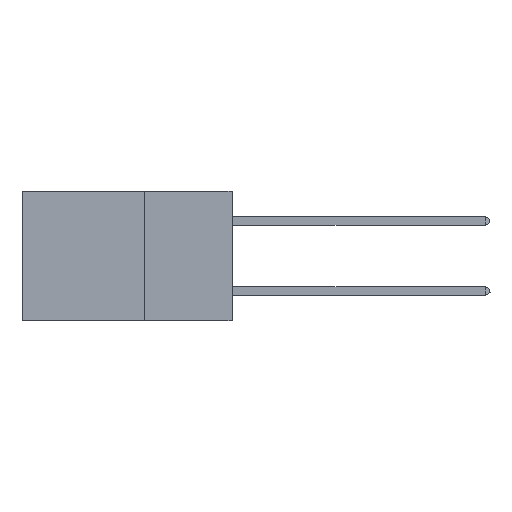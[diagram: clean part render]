
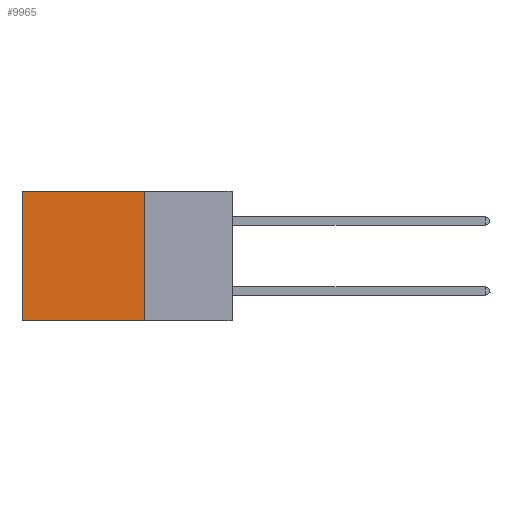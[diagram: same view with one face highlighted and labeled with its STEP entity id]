
A CAD part, left-side view. The second image highlights one B-rep face of the part: STEP entity #9965.
In plain terms, the highlighted planar face has unit normal (-1, 0, 0).
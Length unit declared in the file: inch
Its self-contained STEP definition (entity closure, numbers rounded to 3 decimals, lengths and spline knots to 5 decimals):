
#2030 = CARTESIAN_POINT ( 'NONE',  ( 0.2875, 0.25, -0.37 ) ) ;
#3394 = EDGE_CURVE ( 'NONE', #20159, #12420, #3566, .T. ) ;
#3555 = CARTESIAN_POINT ( 'NONE',  ( 0.2875, 0.25, 0. ) ) ;
#3566 = LINE ( 'NONE', #12758, #24923 ) ;
#4373 = EDGE_CURVE ( 'NONE', #9347, #28542, #22340, .T. ) ;
#5568 = VECTOR ( 'NONE', #29239, 39.37008 ) ;
#5815 = EDGE_CURVE ( 'NONE', #28542, #12420, #25143, .T. ) ;
#6469 = FACE_OUTER_BOUND ( 'NONE', #14280, .T. ) ;
#7150 = LINE ( 'NONE', #3555, #11040 ) ;
#9347 = VERTEX_POINT ( 'NONE', #26755 ) ;
#9965 = ADVANCED_FACE ( 'NONE', ( #6469 ), #13038, .F. ) ;
#10123 = DIRECTION ( 'NONE',  ( 0., 0., -1. ) ) ;
#11040 = VECTOR ( 'NONE', #17330, 39.37008 ) ;
#12118 = DIRECTION ( 'NONE',  ( 0., 0., -1. ) ) ;
#12420 = VERTEX_POINT ( 'NONE', #14339 ) ;
#12758 = CARTESIAN_POINT ( 'NONE',  ( 0.2875, 0.6, 0. ) ) ;
#13038 = PLANE ( 'NONE',  #19581 ) ;
#13644 = CARTESIAN_POINT ( 'NONE',  ( 0.2875, 0.25, 0. ) ) ;
#14280 = EDGE_LOOP ( 'NONE', ( #21266, #21274, #27139, #23926 ) ) ;
#14339 = CARTESIAN_POINT ( 'NONE',  ( 0.2875, 0.6, -0.37 ) ) ;
#14452 = CARTESIAN_POINT ( 'NONE',  ( 0.2875, 0.25, 0. ) ) ;
#15931 = DIRECTION ( 'NONE',  ( 1., 0., 0. ) ) ;
#17330 = DIRECTION ( 'NONE',  ( 0., 1., 0. ) ) ;
#19477 = VECTOR ( 'NONE', #12118, 39.37008 ) ;
#19581 = AXIS2_PLACEMENT_3D ( 'NONE', #13644, #15931, #20782 ) ;
#20159 = VERTEX_POINT ( 'NONE', #23044 ) ;
#20782 = DIRECTION ( 'NONE',  ( 0., 0., -1. ) ) ;
#21266 = ORIENTED_EDGE ( 'NONE', *, *, #3394, .T. ) ;
#21274 = ORIENTED_EDGE ( 'NONE', *, *, #5815, .F. ) ;
#22340 = LINE ( 'NONE', #14452, #19477 ) ;
#23044 = CARTESIAN_POINT ( 'NONE',  ( 0.2875, 0.6, 0. ) ) ;
#23282 = CARTESIAN_POINT ( 'NONE',  ( 0.2875, 0.25, -0.37 ) ) ;
#23926 = ORIENTED_EDGE ( 'NONE', *, *, #26155, .T. ) ;
#24923 = VECTOR ( 'NONE', #10123, 39.37008 ) ;
#25143 = LINE ( 'NONE', #2030, #5568 ) ;
#26155 = EDGE_CURVE ( 'NONE', #9347, #20159, #7150, .T. ) ;
#26755 = CARTESIAN_POINT ( 'NONE',  ( 0.2875, 0.25, 0. ) ) ;
#27139 = ORIENTED_EDGE ( 'NONE', *, *, #4373, .F. ) ;
#28542 = VERTEX_POINT ( 'NONE', #23282 ) ;
#29239 = DIRECTION ( 'NONE',  ( 0., 1., 0. ) ) ;
